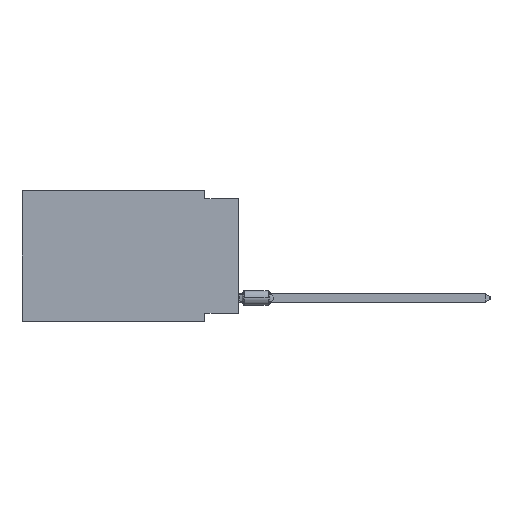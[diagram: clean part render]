
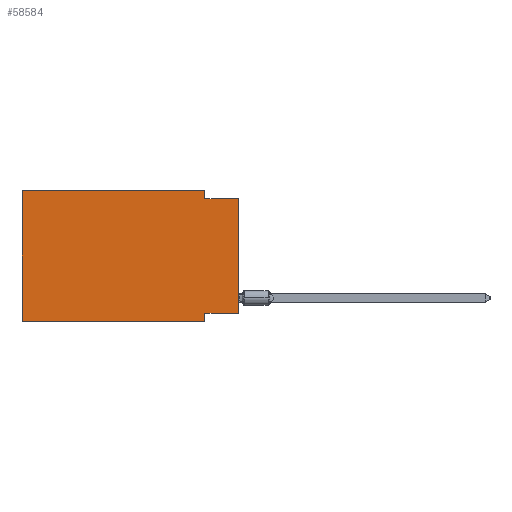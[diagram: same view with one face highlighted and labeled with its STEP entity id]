
A CAD part, left-side view. The second image highlights one B-rep face of the part: STEP entity #58584.
In plain terms, the highlighted planar face has unit normal (-1, 0, 0).
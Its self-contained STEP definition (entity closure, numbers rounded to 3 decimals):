
#2537 = CARTESIAN_POINT ( 'NONE',  ( 0., 16.383, -9.906 ) ) ;
#2921 = DIRECTION ( 'NONE',  ( 0., 0., 1. ) ) ;
#3073 = EDGE_CURVE ( 'NONE', #44122, #3661, #4686, .T. ) ;
#3661 = VERTEX_POINT ( 'NONE', #62038 ) ;
#4594 = LINE ( 'NONE', #53023, #61477 ) ;
#4686 = LINE ( 'NONE', #58334, #42714 ) ;
#4964 = LINE ( 'NONE', #31449, #6306 ) ;
#6123 = FACE_OUTER_BOUND ( 'NONE', #25059, .T. ) ;
#6306 = VECTOR ( 'NONE', #36669, 1000. ) ;
#8249 = EDGE_CURVE ( 'NONE', #32809, #26462, #29394, .T. ) ;
#9165 = CARTESIAN_POINT ( 'NONE',  ( 0., 0., -0.635 ) ) ;
#10124 = VERTEX_POINT ( 'NONE', #67000 ) ;
#13280 = ORIENTED_EDGE ( 'NONE', *, *, #51549, .F. ) ;
#14785 = CARTESIAN_POINT ( 'NONE',  ( 0., 16.383, 0. ) ) ;
#15446 = DIRECTION ( 'NONE',  ( 0., -1., 0. ) ) ;
#16220 = CARTESIAN_POINT ( 'NONE',  ( 0., 16.383, 0. ) ) ;
#17762 = EDGE_CURVE ( 'NONE', #3661, #26462, #40253, .T. ) ;
#18312 = DIRECTION ( 'NONE',  ( 0., -1., 0. ) ) ;
#19075 = VECTOR ( 'NONE', #21241, 1000. ) ;
#20425 = AXIS2_PLACEMENT_3D ( 'NONE', #16220, #37484, #31229 ) ;
#20549 = CARTESIAN_POINT ( 'NONE',  ( 0., 2.54, 0. ) ) ;
#21241 = DIRECTION ( 'NONE',  ( 0., -1., 0. ) ) ;
#22094 = DIRECTION ( 'NONE',  ( 0., 0., -1. ) ) ;
#22230 = ORIENTED_EDGE ( 'NONE', *, *, #8249, .T. ) ;
#25059 = EDGE_LOOP ( 'NONE', ( #22230, #68614, #58731, #13280, #28712, #67836, #44745, #66485 ) ) ;
#26462 = VERTEX_POINT ( 'NONE', #9165 ) ;
#26567 = VECTOR ( 'NONE', #26644, 1000. ) ;
#26589 = EDGE_CURVE ( 'NONE', #32809, #10124, #4964, .T. ) ;
#26644 = DIRECTION ( 'NONE',  ( 0., 0., -1. ) ) ;
#26760 = VERTEX_POINT ( 'NONE', #65602 ) ;
#27524 = CARTESIAN_POINT ( 'NONE',  ( 0., 16.383, -9.906 ) ) ;
#28024 = CARTESIAN_POINT ( 'NONE',  ( 0., 2.54, -9.906 ) ) ;
#28712 = ORIENTED_EDGE ( 'NONE', *, *, #52008, .F. ) ;
#29394 = LINE ( 'NONE', #67050, #33888 ) ;
#31229 = DIRECTION ( 'NONE',  ( 0., 0., -1. ) ) ;
#31413 = DIRECTION ( 'NONE',  ( 0., 0., 1. ) ) ;
#31449 = CARTESIAN_POINT ( 'NONE',  ( 0., 0., -9.271 ) ) ;
#32518 = VECTOR ( 'NONE', #15446, 1000. ) ;
#32809 = VERTEX_POINT ( 'NONE', #42536 ) ;
#33888 = VECTOR ( 'NONE', #2921, 1000. ) ;
#36669 = DIRECTION ( 'NONE',  ( 0., 1., 0. ) ) ;
#37484 = DIRECTION ( 'NONE',  ( 1., 0., 0. ) ) ;
#40253 = LINE ( 'NONE', #66079, #40365 ) ;
#40365 = VECTOR ( 'NONE', #18312, 1000. ) ;
#42536 = CARTESIAN_POINT ( 'NONE',  ( 0., 0., -9.271 ) ) ;
#42714 = VECTOR ( 'NONE', #22094, 1000. ) ;
#44122 = VERTEX_POINT ( 'NONE', #20549 ) ;
#44322 = CARTESIAN_POINT ( 'NONE',  ( 0., 2.54, -9.906 ) ) ;
#44745 = ORIENTED_EDGE ( 'NONE', *, *, #46286, .F. ) ;
#46286 = EDGE_CURVE ( 'NONE', #10124, #46725, #59031, .T. ) ;
#46725 = VERTEX_POINT ( 'NONE', #44322 ) ;
#51549 = EDGE_CURVE ( 'NONE', #26760, #44122, #63557, .T. ) ;
#52008 = EDGE_CURVE ( 'NONE', #59217, #26760, #4594, .T. ) ;
#53023 = CARTESIAN_POINT ( 'NONE',  ( 0., 16.383, 0. ) ) ;
#53650 = LINE ( 'NONE', #27524, #19075 ) ;
#57060 = EDGE_CURVE ( 'NONE', #59217, #46725, #53650, .T. ) ;
#58334 = CARTESIAN_POINT ( 'NONE',  ( 0., 2.54, 0. ) ) ;
#58584 = ADVANCED_FACE ( 'NONE', ( #6123 ), #64684, .F. ) ;
#58731 = ORIENTED_EDGE ( 'NONE', *, *, #3073, .F. ) ;
#59031 = LINE ( 'NONE', #28024, #26567 ) ;
#59217 = VERTEX_POINT ( 'NONE', #2537 ) ;
#61477 = VECTOR ( 'NONE', #31413, 1000. ) ;
#62038 = CARTESIAN_POINT ( 'NONE',  ( 0., 2.54, -0.635 ) ) ;
#63557 = LINE ( 'NONE', #14785, #32518 ) ;
#64684 = PLANE ( 'NONE',  #20425 ) ;
#65602 = CARTESIAN_POINT ( 'NONE',  ( 0., 16.383, 0. ) ) ;
#66079 = CARTESIAN_POINT ( 'NONE',  ( 0., 0., -0.635 ) ) ;
#66485 = ORIENTED_EDGE ( 'NONE', *, *, #26589, .F. ) ;
#67000 = CARTESIAN_POINT ( 'NONE',  ( 0., 2.54, -9.271 ) ) ;
#67050 = CARTESIAN_POINT ( 'NONE',  ( 0., 0., 0. ) ) ;
#67836 = ORIENTED_EDGE ( 'NONE', *, *, #57060, .T. ) ;
#68614 = ORIENTED_EDGE ( 'NONE', *, *, #17762, .F. ) ;
